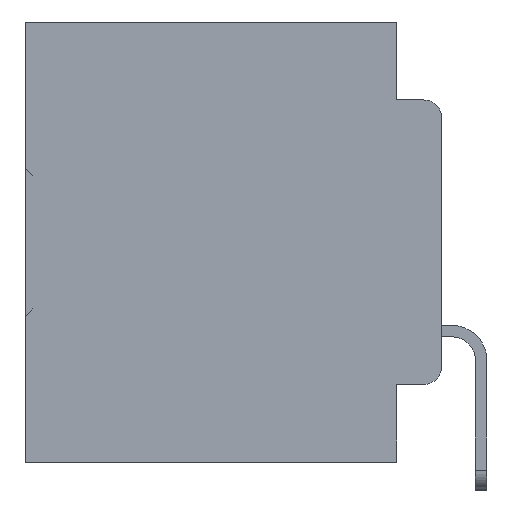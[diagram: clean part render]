
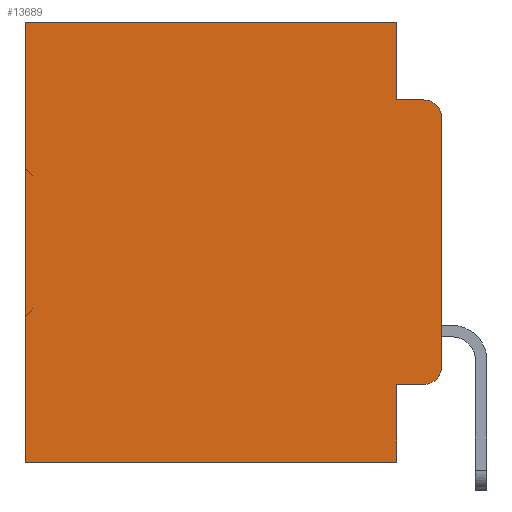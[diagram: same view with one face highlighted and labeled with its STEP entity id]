
A CAD part, left-side view. The second image highlights one B-rep face of the part: STEP entity #13689.
In plain terms, the highlighted planar face has unit normal (-1, 0, 0).
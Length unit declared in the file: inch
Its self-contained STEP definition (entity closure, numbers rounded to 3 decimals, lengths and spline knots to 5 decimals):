
#291 = LINE ( 'NONE', #5172, #34699 ) ;
#453 = ORIENTED_EDGE ( 'NONE', *, *, #20796, .T. ) ;
#797 = DIRECTION ( 'NONE',  ( 0., 0., -1. ) ) ;
#1010 = LINE ( 'NONE', #16445, #25757 ) ;
#2128 = VECTOR ( 'NONE', #26237, 39.37008 ) ;
#3054 = VERTEX_POINT ( 'NONE', #31465 ) ;
#3152 = VERTEX_POINT ( 'NONE', #23761 ) ;
#3251 = EDGE_CURVE ( 'NONE', #11612, #14063, #4926, .T. ) ;
#4583 = VERTEX_POINT ( 'NONE', #26031 ) ;
#4926 = CIRCLE ( 'NONE', #31713, 0.02 ) ;
#5111 = EDGE_LOOP ( 'NONE', ( #27826, #27105, #30965, #19897, #35239, #453, #21342, #11532, #33616, #11872 ) ) ;
#5172 = CARTESIAN_POINT ( 'NONE',  ( 0.298, 0.051, 0. ) ) ;
#6242 = EDGE_CURVE ( 'NONE', #3152, #3054, #291, .T. ) ;
#6434 = DIRECTION ( 'NONE',  ( 0., -1., 0. ) ) ;
#7257 = AXIS2_PLACEMENT_3D ( 'NONE', #37165, #7431, #22430 ) ;
#7424 = VERTEX_POINT ( 'NONE', #13168 ) ;
#7431 = DIRECTION ( 'NONE',  ( 1., 0., 0. ) ) ;
#8220 = CARTESIAN_POINT ( 'NONE',  ( 0.298, 0.02, -0.0885 ) ) ;
#9308 = EDGE_CURVE ( 'NONE', #4583, #11612, #15257, .T. ) ;
#9520 = CARTESIAN_POINT ( 'NONE',  ( 0.298, 0.051, -0.4115 ) ) ;
#10409 = VECTOR ( 'NONE', #33923, 39.37008 ) ;
#11113 = FACE_OUTER_BOUND ( 'NONE', #5111, .T. ) ;
#11291 = DIRECTION ( 'NONE',  ( -1., 0., 0. ) ) ;
#11325 = EDGE_CURVE ( 'NONE', #7424, #14063, #30138, .T. ) ;
#11532 = ORIENTED_EDGE ( 'NONE', *, *, #24262, .F. ) ;
#11612 = VERTEX_POINT ( 'NONE', #30848 ) ;
#11799 = AXIS2_PLACEMENT_3D ( 'NONE', #13266, #36723, #19036 ) ;
#11872 = ORIENTED_EDGE ( 'NONE', *, *, #3251, .T. ) ;
#12056 = VECTOR ( 'NONE', #6434, 39.37008 ) ;
#13168 = CARTESIAN_POINT ( 'NONE',  ( 0.298, 0., -0.1085 ) ) ;
#13266 = CARTESIAN_POINT ( 'NONE',  ( 0.298, 0.02, -0.1085 ) ) ;
#13443 = CARTESIAN_POINT ( 'NONE',  ( 0.298, 0.051, -0.5 ) ) ;
#13689 = ADVANCED_FACE ( 'NONE', ( #11113 ), #34204, .F. ) ;
#13937 = CIRCLE ( 'NONE', #11799, 0.02 ) ;
#14063 = VERTEX_POINT ( 'NONE', #29682 ) ;
#15133 = LINE ( 'NONE', #29913, #31632 ) ;
#15257 = LINE ( 'NONE', #9520, #12056 ) ;
#15535 = VECTOR ( 'NONE', #24767, 39.37008 ) ;
#16445 = CARTESIAN_POINT ( 'NONE',  ( 0.298, 0., -0.5 ) ) ;
#17071 = EDGE_CURVE ( 'NONE', #3054, #25478, #18208, .T. ) ;
#17787 = CARTESIAN_POINT ( 'NONE',  ( 0.298, 0., 0. ) ) ;
#18208 = LINE ( 'NONE', #36757, #10409 ) ;
#18468 = EDGE_CURVE ( 'NONE', #7424, #25478, #13937, .T. ) ;
#18708 = CARTESIAN_POINT ( 'NONE',  ( 0.298, 0.051, 0. ) ) ;
#18828 = DIRECTION ( 'NONE',  ( 0., 0., -1. ) ) ;
#19036 = DIRECTION ( 'NONE',  ( 0., 0., -1. ) ) ;
#19486 = VECTOR ( 'NONE', #18828, 39.37008 ) ;
#19897 = ORIENTED_EDGE ( 'NONE', *, *, #6242, .F. ) ;
#20796 = EDGE_CURVE ( 'NONE', #21621, #23717, #15133, .T. ) ;
#21342 = ORIENTED_EDGE ( 'NONE', *, *, #25457, .F. ) ;
#21621 = VERTEX_POINT ( 'NONE', #31613 ) ;
#22430 = DIRECTION ( 'NONE',  ( 0., 0., -1. ) ) ;
#23717 = VERTEX_POINT ( 'NONE', #33256 ) ;
#23761 = CARTESIAN_POINT ( 'NONE',  ( 0.298, 0.051, 0. ) ) ;
#24262 = EDGE_CURVE ( 'NONE', #4583, #32288, #30047, .T. ) ;
#24767 = DIRECTION ( 'NONE',  ( 0., 1., 0. ) ) ;
#25457 = EDGE_CURVE ( 'NONE', #32288, #23717, #1010, .T. ) ;
#25478 = VERTEX_POINT ( 'NONE', #8220 ) ;
#25633 = CARTESIAN_POINT ( 'NONE',  ( 0.298, 0.02, -0.3915 ) ) ;
#25757 = VECTOR ( 'NONE', #36933, 39.37008 ) ;
#26031 = CARTESIAN_POINT ( 'NONE',  ( 0.298, 0.051, -0.4115 ) ) ;
#26237 = DIRECTION ( 'NONE',  ( 0., 0., -1. ) ) ;
#27105 = ORIENTED_EDGE ( 'NONE', *, *, #18468, .T. ) ;
#27826 = ORIENTED_EDGE ( 'NONE', *, *, #11325, .F. ) ;
#28469 = DIRECTION ( 'NONE',  ( 0., 0., -1. ) ) ;
#29682 = CARTESIAN_POINT ( 'NONE',  ( 0.298, 0., -0.3915 ) ) ;
#29913 = CARTESIAN_POINT ( 'NONE',  ( 0.298, 0.473, 0. ) ) ;
#30047 = LINE ( 'NONE', #18708, #19486 ) ;
#30138 = LINE ( 'NONE', #17787, #2128 ) ;
#30848 = CARTESIAN_POINT ( 'NONE',  ( 0.298, 0.02, -0.4115 ) ) ;
#30932 = DIRECTION ( 'NONE',  ( 0., 0., -1. ) ) ;
#30965 = ORIENTED_EDGE ( 'NONE', *, *, #17071, .F. ) ;
#31465 = CARTESIAN_POINT ( 'NONE',  ( 0.298, 0.051, -0.0885 ) ) ;
#31492 = EDGE_CURVE ( 'NONE', #3152, #21621, #38028, .T. ) ;
#31613 = CARTESIAN_POINT ( 'NONE',  ( 0.298, 0.473, 0. ) ) ;
#31632 = VECTOR ( 'NONE', #797, 39.37008 ) ;
#31713 = AXIS2_PLACEMENT_3D ( 'NONE', #25633, #11291, #28469 ) ;
#32288 = VERTEX_POINT ( 'NONE', #13443 ) ;
#33256 = CARTESIAN_POINT ( 'NONE',  ( 0.298, 0.473, -0.5 ) ) ;
#33371 = CARTESIAN_POINT ( 'NONE',  ( 0.298, 0., 0. ) ) ;
#33616 = ORIENTED_EDGE ( 'NONE', *, *, #9308, .T. ) ;
#33923 = DIRECTION ( 'NONE',  ( 0., -1., 0. ) ) ;
#34204 = PLANE ( 'NONE',  #7257 ) ;
#34699 = VECTOR ( 'NONE', #30932, 39.37008 ) ;
#35239 = ORIENTED_EDGE ( 'NONE', *, *, #31492, .T. ) ;
#36723 = DIRECTION ( 'NONE',  ( -1., 0., 0. ) ) ;
#36757 = CARTESIAN_POINT ( 'NONE',  ( 0.298, 0.051, -0.0885 ) ) ;
#36933 = DIRECTION ( 'NONE',  ( 0., 1., 0. ) ) ;
#37165 = CARTESIAN_POINT ( 'NONE',  ( 0.298, 0., 0. ) ) ;
#38028 = LINE ( 'NONE', #33371, #15535 ) ;
